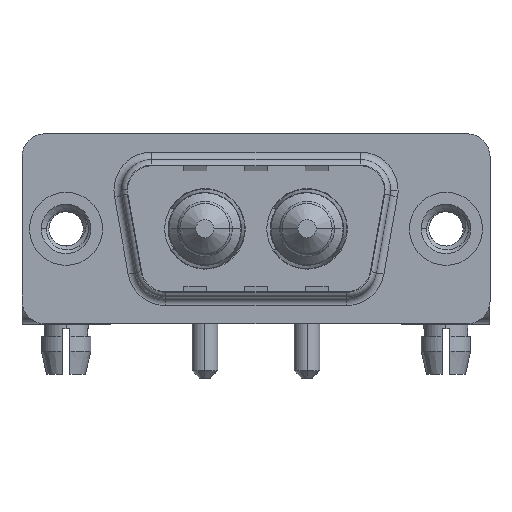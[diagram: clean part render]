
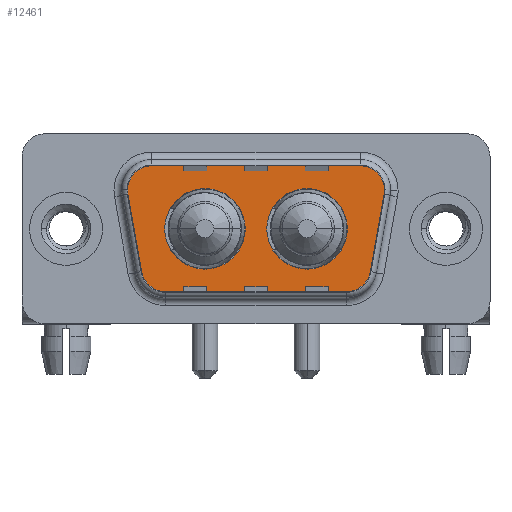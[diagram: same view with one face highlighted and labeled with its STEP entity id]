
A CAD part, top view. The second image highlights one B-rep face of the part: STEP entity #12461.
In plain terms, the highlighted planar face has unit normal (0, 0, 1).
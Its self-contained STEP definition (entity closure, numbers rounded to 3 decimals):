
#46 = DIRECTION ( 'NONE',  ( -1., 0., 0. ) ) ;
#163 = AXIS2_PLACEMENT_3D ( 'NONE', #8474, #2125, #9612 ) ;
#164 = VERTEX_POINT ( 'NONE', #4368 ) ;
#581 = AXIS2_PLACEMENT_3D ( 'NONE', #5730, #5594, #4613 ) ;
#639 = ORIENTED_EDGE ( 'NONE', *, *, #6535, .T. ) ;
#641 = CIRCLE ( 'NONE', #6509, 2. ) ;
#737 = CARTESIAN_POINT ( 'NONE',  ( 18.541, -4.9, 0. ) ) ;
#961 = PLANE ( 'NONE',  #1044 ) ;
#1044 = AXIS2_PLACEMENT_3D ( 'NONE', #1169, #11683, #12816 ) ;
#1138 = DIRECTION ( 'NONE',  ( 0.174, 0.985, 0. ) ) ;
#1169 = CARTESIAN_POINT ( 'NONE',  ( 18.541, -2.9, 0. ) ) ;
#1318 = EDGE_CURVE ( 'NONE', #4944, #2712, #8118, .T. ) ;
#1337 = CARTESIAN_POINT ( 'NONE',  ( 6.459, -2.9, 0. ) ) ;
#1479 = ORIENTED_EDGE ( 'NONE', *, *, #5563, .F. ) ;
#1678 = VERTEX_POINT ( 'NONE', #3819 ) ;
#1732 = VERTEX_POINT ( 'NONE', #3889 ) ;
#1734 = DIRECTION ( 'NONE',  ( 0., 0., 1. ) ) ;
#1905 = EDGE_LOOP ( 'NONE', ( #9115, #1479 ) ) ;
#2010 = LINE ( 'NONE', #7295, #10365 ) ;
#2079 = DIRECTION ( 'NONE',  ( 1., 0., 0. ) ) ;
#2125 = DIRECTION ( 'NONE',  ( 0., 0., 1. ) ) ;
#2422 = CARTESIAN_POINT ( 'NONE',  ( 6.49, 0., 0. ) ) ;
#2712 = VERTEX_POINT ( 'NONE', #2422 ) ;
#2858 = CARTESIAN_POINT ( 'NONE',  ( 11.79, 0., 0. ) ) ;
#3043 = EDGE_CURVE ( 'NONE', #5214, #3610, #11063, .T. ) ;
#3085 = FACE_BOUND ( 'NONE', #1905, .T. ) ;
#3128 = AXIS2_PLACEMENT_3D ( 'NONE', #3777, #12515, #4983 ) ;
#3165 = EDGE_CURVE ( 'NONE', #6366, #12456, #9497, .T. ) ;
#3291 = ORIENTED_EDGE ( 'NONE', *, *, #7643, .T. ) ;
#3405 = AXIS2_PLACEMENT_3D ( 'NONE', #12471, #3940, #9234 ) ;
#3571 = EDGE_CURVE ( 'NONE', #12997, #7548, #4435, .T. ) ;
#3610 = VERTEX_POINT ( 'NONE', #11188 ) ;
#3745 = EDGE_CURVE ( 'NONE', #7548, #5205, #10512, .T. ) ;
#3777 = CARTESIAN_POINT ( 'NONE',  ( 19.564, 2.9, 0. ) ) ;
#3819 = CARTESIAN_POINT ( 'NONE',  ( 6.459, -4.9, 0. ) ) ;
#3889 = CARTESIAN_POINT ( 'NONE',  ( 21.564, 2.9, 0. ) ) ;
#3940 = DIRECTION ( 'NONE',  ( 0., 0., 1. ) ) ;
#4368 = CARTESIAN_POINT ( 'NONE',  ( 21.534, 2.553, 0. ) ) ;
#4413 = EDGE_LOOP ( 'NONE', ( #6890, #12409, #4780, #6211, #9725, #6832, #3291, #13199, #639 ) ) ;
#4435 = LINE ( 'NONE', #10973, #7131 ) ;
#4457 = DIRECTION ( 'NONE',  ( 0., 0., 1. ) ) ;
#4563 = CARTESIAN_POINT ( 'NONE',  ( 9.14, 0., 0. ) ) ;
#4583 = DIRECTION ( 'NONE',  ( 0., 0., 1. ) ) ;
#4613 = DIRECTION ( 'NONE',  ( -1., 0., 0. ) ) ;
#4734 = VECTOR ( 'NONE', #6561, 1000. ) ;
#4780 = ORIENTED_EDGE ( 'NONE', *, *, #10073, .T. ) ;
#4944 = VERTEX_POINT ( 'NONE', #2858 ) ;
#4955 = EDGE_CURVE ( 'NONE', #1732, #12997, #12123, .T. ) ;
#4983 = DIRECTION ( 'NONE',  ( -1., 0., 0. ) ) ;
#5205 = VERTEX_POINT ( 'NONE', #9699 ) ;
#5214 = VERTEX_POINT ( 'NONE', #10682 ) ;
#5262 = VERTEX_POINT ( 'NONE', #10876 ) ;
#5315 = EDGE_LOOP ( 'NONE', ( #9837, #11051 ) ) ;
#5347 = DIRECTION ( 'NONE',  ( 0., 0., 1. ) ) ;
#5563 = EDGE_CURVE ( 'NONE', #2712, #4944, #11655, .T. ) ;
#5594 = DIRECTION ( 'NONE',  ( 0., 0., 1. ) ) ;
#5696 = CARTESIAN_POINT ( 'NONE',  ( 3.466, 2.553, 0. ) ) ;
#5729 = CARTESIAN_POINT ( 'NONE',  ( 15.86, 0., 0. ) ) ;
#5730 = CARTESIAN_POINT ( 'NONE',  ( 19.564, 2.9, 0. ) ) ;
#6211 = ORIENTED_EDGE ( 'NONE', *, *, #4955, .T. ) ;
#6366 = VERTEX_POINT ( 'NONE', #737 ) ;
#6448 = VECTOR ( 'NONE', #1138, 1000. ) ;
#6509 = AXIS2_PLACEMENT_3D ( 'NONE', #1337, #4457, #8750 ) ;
#6535 = EDGE_CURVE ( 'NONE', #1678, #6366, #2010, .T. ) ;
#6561 = DIRECTION ( 'NONE',  ( 0.174, -0.985, 0. ) ) ;
#6810 = EDGE_CURVE ( 'NONE', #3610, #5214, #12410, .T. ) ;
#6822 = CARTESIAN_POINT ( 'NONE',  ( 15.86, 0., 0. ) ) ;
#6832 = ORIENTED_EDGE ( 'NONE', *, *, #3745, .T. ) ;
#6890 = ORIENTED_EDGE ( 'NONE', *, *, #3165, .T. ) ;
#7131 = VECTOR ( 'NONE', #46, 1000. ) ;
#7295 = CARTESIAN_POINT ( 'NONE',  ( 6.459, -4.9, 0. ) ) ;
#7341 = CIRCLE ( 'NONE', #581, 2. ) ;
#7409 = CARTESIAN_POINT ( 'NONE',  ( 5.436, 4.9, 0. ) ) ;
#7458 = FACE_BOUND ( 'NONE', #5315, .T. ) ;
#7548 = VERTEX_POINT ( 'NONE', #7409 ) ;
#7643 = EDGE_CURVE ( 'NONE', #5205, #5262, #8872, .T. ) ;
#7918 = DIRECTION ( 'NONE',  ( 0., 0., 1. ) ) ;
#8118 = CIRCLE ( 'NONE', #8576, 2.65 ) ;
#8357 = AXIS2_PLACEMENT_3D ( 'NONE', #6822, #4583, #10082 ) ;
#8362 = DIRECTION ( 'NONE',  ( 1., 0., 0. ) ) ;
#8474 = CARTESIAN_POINT ( 'NONE',  ( 9.14, 0., 0. ) ) ;
#8576 = AXIS2_PLACEMENT_3D ( 'NONE', #4563, #5347, #12817 ) ;
#8724 = CARTESIAN_POINT ( 'NONE',  ( 20.511, -3.247, 0. ) ) ;
#8750 = DIRECTION ( 'NONE',  ( -1., 0., 0. ) ) ;
#8804 = AXIS2_PLACEMENT_3D ( 'NONE', #5729, #7918, #12078 ) ;
#8872 = LINE ( 'NONE', #5696, #4734 ) ;
#8918 = EDGE_CURVE ( 'NONE', #12456, #164, #12707, .T. ) ;
#9115 = ORIENTED_EDGE ( 'NONE', *, *, #1318, .F. ) ;
#9234 = DIRECTION ( 'NONE',  ( 1., 0., 0. ) ) ;
#9497 = CIRCLE ( 'NONE', #3405, 2. ) ;
#9612 = DIRECTION ( 'NONE',  ( 1., 0., 0. ) ) ;
#9699 = CARTESIAN_POINT ( 'NONE',  ( 3.466, 2.553, 0. ) ) ;
#9725 = ORIENTED_EDGE ( 'NONE', *, *, #3571, .T. ) ;
#9837 = ORIENTED_EDGE ( 'NONE', *, *, #6810, .F. ) ;
#10073 = EDGE_CURVE ( 'NONE', #164, #1732, #7341, .T. ) ;
#10082 = DIRECTION ( 'NONE',  ( 1., 0., 0. ) ) ;
#10365 = VECTOR ( 'NONE', #2079, 1000. ) ;
#10512 = CIRCLE ( 'NONE', #12079, 2. ) ;
#10682 = CARTESIAN_POINT ( 'NONE',  ( 13.21, 0., 0. ) ) ;
#10803 = CARTESIAN_POINT ( 'NONE',  ( 21.534, 2.553, 0. ) ) ;
#10838 = FACE_OUTER_BOUND ( 'NONE', #4413, .T. ) ;
#10876 = CARTESIAN_POINT ( 'NONE',  ( 4.489, -3.247, 0. ) ) ;
#10973 = CARTESIAN_POINT ( 'NONE',  ( 5.436, 4.9, 0. ) ) ;
#11051 = ORIENTED_EDGE ( 'NONE', *, *, #3043, .F. ) ;
#11063 = CIRCLE ( 'NONE', #8357, 2.65 ) ;
#11188 = CARTESIAN_POINT ( 'NONE',  ( 18.51, 0., 0. ) ) ;
#11396 = CARTESIAN_POINT ( 'NONE',  ( 5.436, 2.9, 0. ) ) ;
#11655 = CIRCLE ( 'NONE', #163, 2.65 ) ;
#11683 = DIRECTION ( 'NONE',  ( 0., 0., 1. ) ) ;
#12078 = DIRECTION ( 'NONE',  ( 1., 0., 0. ) ) ;
#12079 = AXIS2_PLACEMENT_3D ( 'NONE', #11396, #1734, #8362 ) ;
#12123 = CIRCLE ( 'NONE', #3128, 2. ) ;
#12409 = ORIENTED_EDGE ( 'NONE', *, *, #8918, .T. ) ;
#12410 = CIRCLE ( 'NONE', #8804, 2.65 ) ;
#12456 = VERTEX_POINT ( 'NONE', #8724 ) ;
#12461 = ADVANCED_FACE ( 'NONE', ( #7458, #3085, #10838 ), #961, .T. ) ;
#12471 = CARTESIAN_POINT ( 'NONE',  ( 18.541, -2.9, 0. ) ) ;
#12515 = DIRECTION ( 'NONE',  ( 0., 0., 1. ) ) ;
#12656 = CARTESIAN_POINT ( 'NONE',  ( 19.564, 4.9, 0. ) ) ;
#12707 = LINE ( 'NONE', #10803, #6448 ) ;
#12816 = DIRECTION ( 'NONE',  ( 1., 0., 0. ) ) ;
#12817 = DIRECTION ( 'NONE',  ( 1., 0., 0. ) ) ;
#12997 = VERTEX_POINT ( 'NONE', #12656 ) ;
#13199 = ORIENTED_EDGE ( 'NONE', *, *, #13912, .T. ) ;
#13912 = EDGE_CURVE ( 'NONE', #5262, #1678, #641, .T. ) ;
